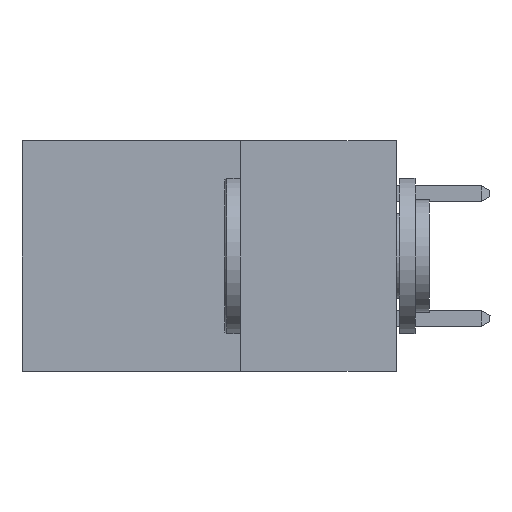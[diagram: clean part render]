
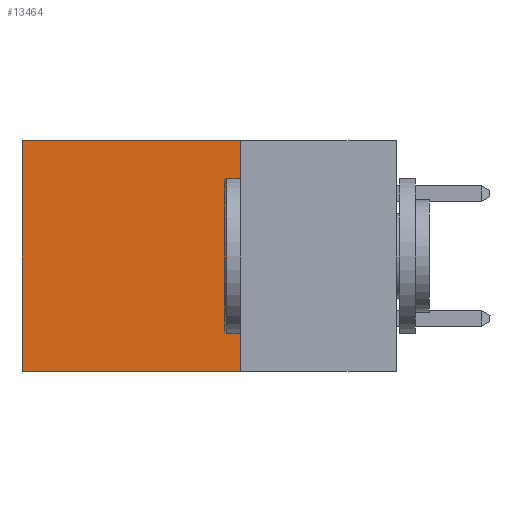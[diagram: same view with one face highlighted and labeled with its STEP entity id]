
A CAD part, left-side view. The second image highlights one B-rep face of the part: STEP entity #13464.
In plain terms, the highlighted planar face has unit normal (-1, 0, 0).
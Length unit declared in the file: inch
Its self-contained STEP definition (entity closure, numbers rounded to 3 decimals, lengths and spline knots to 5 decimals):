
#204 = EDGE_CURVE ( 'NONE', #9273, #16557, #10392, .T. ) ;
#542 = FACE_OUTER_BOUND ( 'NONE', #5250, .T. ) ;
#1459 = CARTESIAN_POINT ( 'NONE',  ( 0.2615, 0.6, -0.37 ) ) ;
#1890 = EDGE_CURVE ( 'NONE', #19835, #6685, #11059, .T. ) ;
#2052 = DIRECTION ( 'NONE',  ( 0., 1., 0. ) ) ;
#3097 = DIRECTION ( 'NONE',  ( 0., 1., 0. ) ) ;
#4847 = CARTESIAN_POINT ( 'NONE',  ( 0.2615, 0.25, -0.37 ) ) ;
#5149 = CARTESIAN_POINT ( 'NONE',  ( 0.2615, 0.25, -0.37 ) ) ;
#5250 = EDGE_LOOP ( 'NONE', ( #8016, #6771, #17786, #11804 ) ) ;
#5841 = VECTOR ( 'NONE', #3097, 39.37008 ) ;
#6154 = VECTOR ( 'NONE', #18761, 39.37008 ) ;
#6425 = DIRECTION ( 'NONE',  ( 0., 0., -1. ) ) ;
#6685 = VERTEX_POINT ( 'NONE', #5149 ) ;
#6732 = EDGE_CURVE ( 'NONE', #19835, #9273, #12862, .T. ) ;
#6771 = ORIENTED_EDGE ( 'NONE', *, *, #19824, .F. ) ;
#8016 = ORIENTED_EDGE ( 'NONE', *, *, #204, .T. ) ;
#8671 = VECTOR ( 'NONE', #2052, 39.37008 ) ;
#9273 = VERTEX_POINT ( 'NONE', #13083 ) ;
#10392 = LINE ( 'NONE', #12391, #6154 ) ;
#11059 = LINE ( 'NONE', #13433, #14735 ) ;
#11135 = CARTESIAN_POINT ( 'NONE',  ( 0.2615, 0.25, -0.37 ) ) ;
#11539 = DIRECTION ( 'NONE',  ( 0., 0., -1. ) ) ;
#11804 = ORIENTED_EDGE ( 'NONE', *, *, #6732, .T. ) ;
#12391 = CARTESIAN_POINT ( 'NONE',  ( 0.2615, 0.6, -0.37 ) ) ;
#12741 = CARTESIAN_POINT ( 'NONE',  ( 0.2615, 0.25, 0. ) ) ;
#12862 = LINE ( 'NONE', #13169, #8671 ) ;
#13083 = CARTESIAN_POINT ( 'NONE',  ( 0.2615, 0.6, 0. ) ) ;
#13169 = CARTESIAN_POINT ( 'NONE',  ( 0.2615, 0.25, 0. ) ) ;
#13433 = CARTESIAN_POINT ( 'NONE',  ( 0.2615, 0.25, -0.37 ) ) ;
#13464 = ADVANCED_FACE ( 'NONE', ( #542 ), #14312, .F. ) ;
#14257 = LINE ( 'NONE', #11135, #5841 ) ;
#14312 = PLANE ( 'NONE',  #19414 ) ;
#14735 = VECTOR ( 'NONE', #11539, 39.37008 ) ;
#15844 = DIRECTION ( 'NONE',  ( 1., 0., 0. ) ) ;
#16557 = VERTEX_POINT ( 'NONE', #1459 ) ;
#17786 = ORIENTED_EDGE ( 'NONE', *, *, #1890, .F. ) ;
#18761 = DIRECTION ( 'NONE',  ( 0., 0., -1. ) ) ;
#19414 = AXIS2_PLACEMENT_3D ( 'NONE', #4847, #15844, #6425 ) ;
#19824 = EDGE_CURVE ( 'NONE', #6685, #16557, #14257, .T. ) ;
#19835 = VERTEX_POINT ( 'NONE', #12741 ) ;
